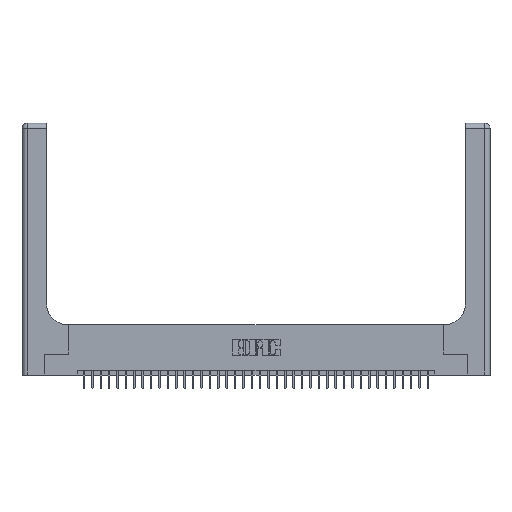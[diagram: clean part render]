
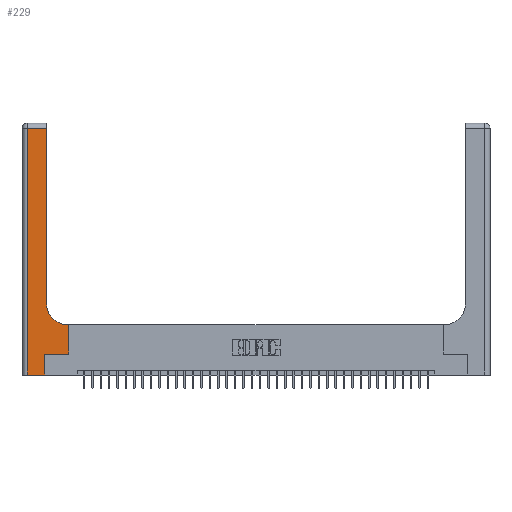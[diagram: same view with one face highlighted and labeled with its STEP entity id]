
A CAD part, top view. The second image highlights one B-rep face of the part: STEP entity #229.
In plain terms, the highlighted planar face has unit normal (0, 0, 1).
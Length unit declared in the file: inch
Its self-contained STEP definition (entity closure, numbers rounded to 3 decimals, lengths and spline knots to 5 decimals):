
#40 = ORIENTED_EDGE ( 'NONE', *, *, #21893, .T. ) ;
#229 = ADVANCED_FACE ( 'NONE', ( #36583 ), #13497, .F. ) ;
#1396 = EDGE_CURVE ( 'NONE', #15082, #29306, #26832, .T. ) ;
#1686 = ORIENTED_EDGE ( 'NONE', *, *, #27666, .T. ) ;
#1688 = VERTEX_POINT ( 'NONE', #37057 ) ;
#2365 = CARTESIAN_POINT ( 'NONE',  ( 0.269, 0.25, 0.37 ) ) ;
#3009 = LINE ( 'NONE', #3678, #20161 ) ;
#3067 = DIRECTION ( 'NONE',  ( 1., 0., 0. ) ) ;
#3146 = VERTEX_POINT ( 'NONE', #18802 ) ;
#3430 = EDGE_CURVE ( 'NONE', #15313, #36581, #6770, .T. ) ;
#3678 = CARTESIAN_POINT ( 'NONE',  ( 0., 2.94, 0.37 ) ) ;
#4659 = CARTESIAN_POINT ( 'NONE',  ( 0., 3., 0.37 ) ) ;
#5617 = LINE ( 'NONE', #24595, #28323 ) ;
#6770 = LINE ( 'NONE', #27888, #14701 ) ;
#7125 = ORIENTED_EDGE ( 'NONE', *, *, #37756, .T. ) ;
#7492 = DIRECTION ( 'NONE',  ( -1., 0., 0. ) ) ;
#7596 = ORIENTED_EDGE ( 'NONE', *, *, #17783, .T. ) ;
#8750 = VECTOR ( 'NONE', #24744, 39.37008 ) ;
#9121 = AXIS2_PLACEMENT_3D ( 'NONE', #4659, #19703, #7492 ) ;
#9973 = CARTESIAN_POINT ( 'NONE',  ( 0.06, 3., 0.37 ) ) ;
#10440 = DIRECTION ( 'NONE',  ( 1., 0., 0. ) ) ;
#10597 = CARTESIAN_POINT ( 'NONE',  ( 0.5415, 0.85, 0.37 ) ) ;
#10699 = CARTESIAN_POINT ( 'NONE',  ( 0.5415, 0.6, 0.37 ) ) ;
#10984 = VECTOR ( 'NONE', #25158, 39.37008 ) ;
#11573 = LINE ( 'NONE', #9973, #8750 ) ;
#12281 = VERTEX_POINT ( 'NONE', #34420 ) ;
#12365 = CARTESIAN_POINT ( 'NONE',  ( 0.5585, 0.25, 0.37 ) ) ;
#13497 = PLANE ( 'NONE',  #9121 ) ;
#14034 = CARTESIAN_POINT ( 'NONE',  ( 0.2915, 0.85, 0.37 ) ) ;
#14701 = VECTOR ( 'NONE', #28420, 39.37008 ) ;
#15082 = VERTEX_POINT ( 'NONE', #10699 ) ;
#15313 = VERTEX_POINT ( 'NONE', #2365 ) ;
#15399 = CARTESIAN_POINT ( 'NONE',  ( 0.2915, 3., 0.37 ) ) ;
#16263 = VECTOR ( 'NONE', #21163, 39.37008 ) ;
#17783 = EDGE_CURVE ( 'NONE', #12281, #22644, #3009, .T. ) ;
#18802 = CARTESIAN_POINT ( 'NONE',  ( 0.06, 0., 0.37 ) ) ;
#18853 = LINE ( 'NONE', #27737, #10984 ) ;
#19703 = DIRECTION ( 'NONE',  ( 0., 0., -1. ) ) ;
#19970 = ORIENTED_EDGE ( 'NONE', *, *, #3430, .T. ) ;
#20161 = VECTOR ( 'NONE', #29611, 39.37008 ) ;
#21163 = DIRECTION ( 'NONE',  ( -1., 0., 0. ) ) ;
#21289 = EDGE_LOOP ( 'NONE', ( #7125, #7596, #34180, #21793, #37713, #19970, #1686, #40, #35835 ) ) ;
#21793 = ORIENTED_EDGE ( 'NONE', *, *, #31132, .T. ) ;
#21893 = EDGE_CURVE ( 'NONE', #1688, #15082, #29234, .T. ) ;
#22644 = VERTEX_POINT ( 'NONE', #32998 ) ;
#22758 = EDGE_CURVE ( 'NONE', #22644, #3146, #11573, .T. ) ;
#23286 = CARTESIAN_POINT ( 'NONE',  ( 0., 0., 0.37 ) ) ;
#24595 = CARTESIAN_POINT ( 'NONE',  ( 0.5585, 0.25, 0.37 ) ) ;
#24744 = DIRECTION ( 'NONE',  ( 0., -1., 0. ) ) ;
#25026 = EDGE_CURVE ( 'NONE', #35041, #15313, #18853, .T. ) ;
#25158 = DIRECTION ( 'NONE',  ( 0., 1., 0. ) ) ;
#26194 = VECTOR ( 'NONE', #3067, 39.37008 ) ;
#26832 = CIRCLE ( 'NONE', #33426, 0.25 ) ;
#27298 = DIRECTION ( 'NONE',  ( 0., 1., 0. ) ) ;
#27666 = EDGE_CURVE ( 'NONE', #36581, #1688, #5617, .T. ) ;
#27737 = CARTESIAN_POINT ( 'NONE',  ( 0.269, 0., 0.37 ) ) ;
#27888 = CARTESIAN_POINT ( 'NONE',  ( 0.269, 0.25, 0.37 ) ) ;
#28323 = VECTOR ( 'NONE', #33099, 39.37008 ) ;
#28420 = DIRECTION ( 'NONE',  ( 1., 0., 0. ) ) ;
#29146 = DIRECTION ( 'NONE',  ( 0., 0., -1. ) ) ;
#29234 = LINE ( 'NONE', #35610, #16263 ) ;
#29306 = VERTEX_POINT ( 'NONE', #14034 ) ;
#29611 = DIRECTION ( 'NONE',  ( -1., 0., 0. ) ) ;
#30669 = CARTESIAN_POINT ( 'NONE',  ( 0.269, 0., 0.37 ) ) ;
#31010 = LINE ( 'NONE', #15399, #34245 ) ;
#31132 = EDGE_CURVE ( 'NONE', #3146, #35041, #36731, .T. ) ;
#32998 = CARTESIAN_POINT ( 'NONE',  ( 0.06, 2.94, 0.37 ) ) ;
#33099 = DIRECTION ( 'NONE',  ( 0., 1., 0. ) ) ;
#33426 = AXIS2_PLACEMENT_3D ( 'NONE', #10597, #29146, #10440 ) ;
#34180 = ORIENTED_EDGE ( 'NONE', *, *, #22758, .T. ) ;
#34245 = VECTOR ( 'NONE', #27298, 39.37008 ) ;
#34420 = CARTESIAN_POINT ( 'NONE',  ( 0.2915, 2.94, 0.37 ) ) ;
#35041 = VERTEX_POINT ( 'NONE', #30669 ) ;
#35610 = CARTESIAN_POINT ( 'NONE',  ( 0.2915, 0.6, 0.37 ) ) ;
#35835 = ORIENTED_EDGE ( 'NONE', *, *, #1396, .T. ) ;
#36581 = VERTEX_POINT ( 'NONE', #12365 ) ;
#36583 = FACE_OUTER_BOUND ( 'NONE', #21289, .T. ) ;
#36731 = LINE ( 'NONE', #23286, #26194 ) ;
#37057 = CARTESIAN_POINT ( 'NONE',  ( 0.5585, 0.6, 0.37 ) ) ;
#37713 = ORIENTED_EDGE ( 'NONE', *, *, #25026, .T. ) ;
#37756 = EDGE_CURVE ( 'NONE', #29306, #12281, #31010, .T. ) ;
